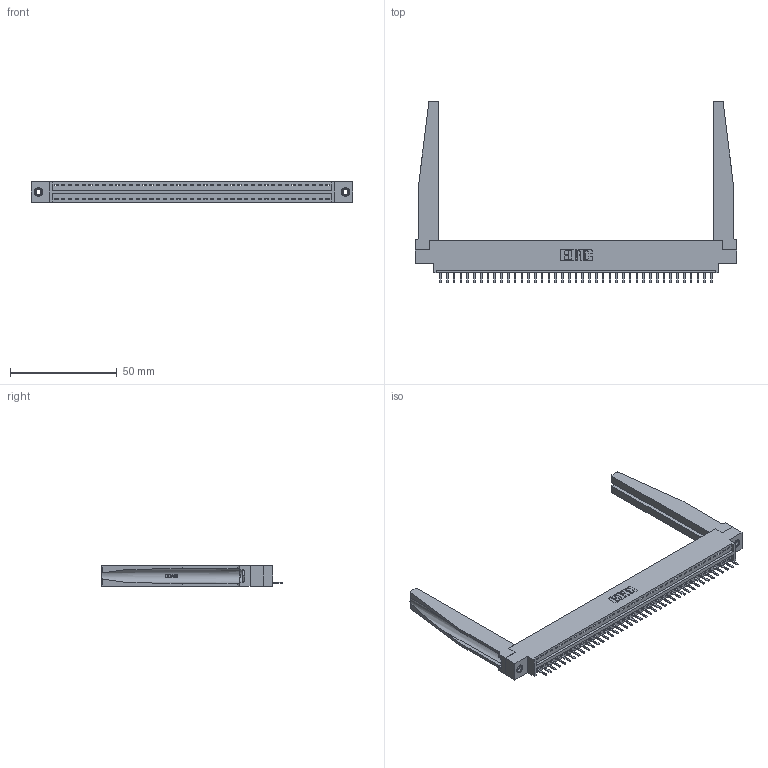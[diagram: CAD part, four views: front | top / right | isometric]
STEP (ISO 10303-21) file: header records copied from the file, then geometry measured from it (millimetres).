
FILE_DESCRIPTION (( 'STEP AP203' ), '1' );
FILE_NAME ('346-041-520-678.STEP', '2022-05-07T11:17:06', ( '' ), ( '' ), 'SwSTEP 2.0', 'SolidWorks 2020', '' );
FILE_SCHEMA (( 'CONFIG_CONTROL_DESIGN' ));
Length unit declared in the file: inch
Products named in the file (5): 346-220-078_345-220-078; 345-250-001_345-250-001-102; 345-292-001_345-293-120; 346 Part_0.170 Offset - 0.156 Dia-TH; 346-041-520-678
Assembly tree (46 placements, depth 2):
  346-041-520-678
    346 Part_0.170 Offset - 0.156 Dia-TH
    345-292-001_345-293-120  x41
    346-220-078_345-220-078  x2
    345-250-001_345-250-001-102  x2
Bounding box: 150.75 x 85.29 x 9.4 mm (x, y, z)
Volume: 21041.3 mm3; surface area: 23992 mm2
Topology: 46 solids, 46 shells, 2916 faces, 8529 edges, 5566 vertices
Faces by surface type: plane 1958, cylinder 906, bspline 36, cone 12, torus 4
Entity records: 30990 total; most frequent: CARTESIAN_POINT 6240, ORIENTED_EDGE 5090, DIRECTION 4477, EDGE_CURVE 2545, LINE 2151, VECTOR 2151, VERTEX_POINT 1688, AXIS2_PLACEMENT_3D 1163
